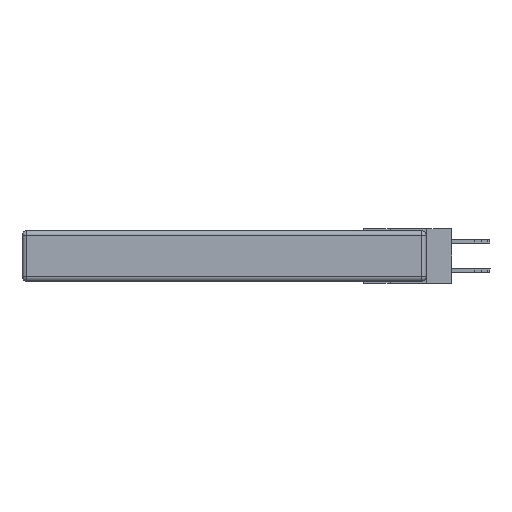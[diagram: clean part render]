
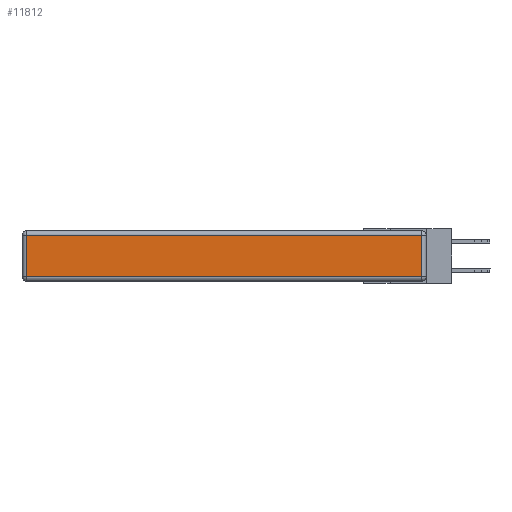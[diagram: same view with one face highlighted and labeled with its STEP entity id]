
A CAD part, left-side view. The second image highlights one B-rep face of the part: STEP entity #11812.
In plain terms, the highlighted planar face has unit normal (-1, 0, 0).
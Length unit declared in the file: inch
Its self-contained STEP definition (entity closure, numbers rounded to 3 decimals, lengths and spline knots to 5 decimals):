
#289 = ORIENTED_EDGE ( 'NONE', *, *, #967, .T. ) ;
#482 = ORIENTED_EDGE ( 'NONE', *, *, #10669, .T. ) ;
#945 = CARTESIAN_POINT ( 'NONE',  ( 0., 0.03, -0.03 ) ) ;
#967 = EDGE_CURVE ( 'NONE', #4471, #14421, #6268, .T. ) ;
#1268 = DIRECTION ( 'NONE',  ( 0., 0., -1. ) ) ;
#1280 = LINE ( 'NONE', #4343, #14599 ) ;
#1693 = CARTESIAN_POINT ( 'NONE',  ( 0., 0.03, -0.343 ) ) ;
#2155 = EDGE_CURVE ( 'NONE', #8186, #4471, #10464, .T. ) ;
#2231 = DIRECTION ( 'NONE',  ( 0., 1., 0. ) ) ;
#2991 = EDGE_LOOP ( 'NONE', ( #289, #482, #13241, #11139 ) ) ;
#3508 = AXIS2_PLACEMENT_3D ( 'NONE', #4888, #15176, #5058 ) ;
#4343 = CARTESIAN_POINT ( 'NONE',  ( 0., 2.75, -0.03 ) ) ;
#4471 = VERTEX_POINT ( 'NONE', #15479 ) ;
#4652 = DIRECTION ( 'NONE',  ( 0., -1., 0. ) ) ;
#4888 = CARTESIAN_POINT ( 'NONE',  ( 0., 0., -0.343 ) ) ;
#5058 = DIRECTION ( 'NONE',  ( 0., 0., 1. ) ) ;
#6184 = PLANE ( 'NONE',  #3508 ) ;
#6268 = LINE ( 'NONE', #16291, #16132 ) ;
#6513 = CARTESIAN_POINT ( 'NONE',  ( 0., 0.03, -0.313 ) ) ;
#7287 = VECTOR ( 'NONE', #13296, 39.37008 ) ;
#7553 = VERTEX_POINT ( 'NONE', #945 ) ;
#8186 = VERTEX_POINT ( 'NONE', #11747 ) ;
#10464 = LINE ( 'NONE', #12811, #11435 ) ;
#10669 = EDGE_CURVE ( 'NONE', #14421, #7553, #14583, .T. ) ;
#11139 = ORIENTED_EDGE ( 'NONE', *, *, #2155, .T. ) ;
#11435 = VECTOR ( 'NONE', #1268, 39.37008 ) ;
#11747 = CARTESIAN_POINT ( 'NONE',  ( 0., 2.72, -0.03 ) ) ;
#11812 = ADVANCED_FACE ( 'NONE', ( #12552 ), #6184, .T. ) ;
#12552 = FACE_OUTER_BOUND ( 'NONE', #2991, .T. ) ;
#12811 = CARTESIAN_POINT ( 'NONE',  ( 0., 2.72, -0.343 ) ) ;
#13241 = ORIENTED_EDGE ( 'NONE', *, *, #16609, .T. ) ;
#13296 = DIRECTION ( 'NONE',  ( 0., 0., 1. ) ) ;
#14421 = VERTEX_POINT ( 'NONE', #6513 ) ;
#14583 = LINE ( 'NONE', #1693, #7287 ) ;
#14599 = VECTOR ( 'NONE', #2231, 39.37008 ) ;
#15176 = DIRECTION ( 'NONE',  ( -1., 0., 0. ) ) ;
#15479 = CARTESIAN_POINT ( 'NONE',  ( 0., 2.72, -0.313 ) ) ;
#16132 = VECTOR ( 'NONE', #4652, 39.37008 ) ;
#16291 = CARTESIAN_POINT ( 'NONE',  ( 0., 0., -0.313 ) ) ;
#16609 = EDGE_CURVE ( 'NONE', #7553, #8186, #1280, .T. ) ;
